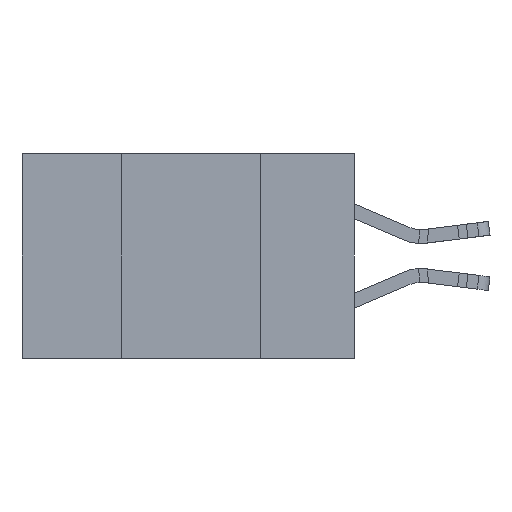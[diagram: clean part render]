
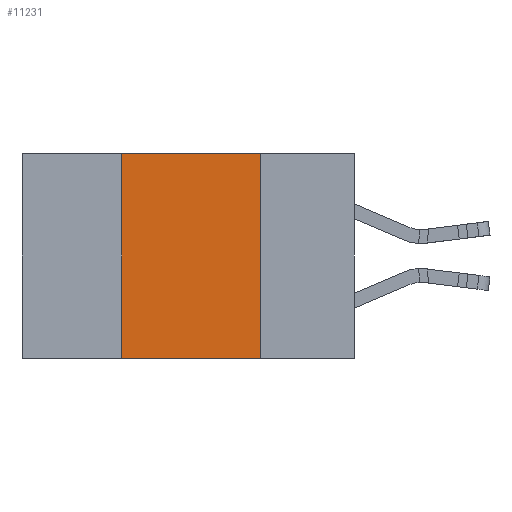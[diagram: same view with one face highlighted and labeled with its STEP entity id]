
A CAD part, left-side view. The second image highlights one B-rep face of the part: STEP entity #11231.
In plain terms, the highlighted planar face has unit normal (-1, 0, 0).
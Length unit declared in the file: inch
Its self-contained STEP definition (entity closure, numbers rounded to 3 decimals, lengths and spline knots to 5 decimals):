
#298 = ORIENTED_EDGE ( 'NONE', *, *, #9223, .T. ) ;
#369 = CARTESIAN_POINT ( 'NONE',  ( 0., 0.42, -0.37 ) ) ;
#645 = CARTESIAN_POINT ( 'NONE',  ( 0., 0.6, -0.37 ) ) ;
#2276 = VECTOR ( 'NONE', #17436, 39.37008 ) ;
#2547 = EDGE_CURVE ( 'NONE', #14172, #7647, #21391, .T. ) ;
#2698 = VERTEX_POINT ( 'NONE', #369 ) ;
#3927 = EDGE_CURVE ( 'NONE', #15790, #14172, #23972, .T. ) ;
#4659 = ORIENTED_EDGE ( 'NONE', *, *, #2547, .F. ) ;
#5021 = ORIENTED_EDGE ( 'NONE', *, *, #13485, .F. ) ;
#5457 = DIRECTION ( 'NONE',  ( 1., 0., 0. ) ) ;
#7014 = FACE_OUTER_BOUND ( 'NONE', #19034, .T. ) ;
#7462 = ORIENTED_EDGE ( 'NONE', *, *, #3927, .F. ) ;
#7647 = VERTEX_POINT ( 'NONE', #14133 ) ;
#9033 = LINE ( 'NONE', #645, #12947 ) ;
#9223 = EDGE_CURVE ( 'NONE', #2698, #7647, #9033, .T. ) ;
#11231 = ADVANCED_FACE ( 'NONE', ( #7014 ), #13076, .F. ) ;
#12184 = AXIS2_PLACEMENT_3D ( 'NONE', #18988, #5457, #16800 ) ;
#12947 = VECTOR ( 'NONE', #22443, 39.37008 ) ;
#13076 = PLANE ( 'NONE',  #12184 ) ;
#13485 = EDGE_CURVE ( 'NONE', #2698, #15790, #15013, .T. ) ;
#14133 = CARTESIAN_POINT ( 'NONE',  ( 0., 0.17, -0.37 ) ) ;
#14172 = VERTEX_POINT ( 'NONE', #25130 ) ;
#15013 = LINE ( 'NONE', #20903, #15773 ) ;
#15773 = VECTOR ( 'NONE', #21032, 39.37008 ) ;
#15790 = VERTEX_POINT ( 'NONE', #24601 ) ;
#16800 = DIRECTION ( 'NONE',  ( 0., 0., -1. ) ) ;
#17436 = DIRECTION ( 'NONE',  ( 0., 0., -1. ) ) ;
#17557 = CARTESIAN_POINT ( 'NONE',  ( 0., 0.17, -0.37 ) ) ;
#18054 = DIRECTION ( 'NONE',  ( 0., -1., 0. ) ) ;
#18988 = CARTESIAN_POINT ( 'NONE',  ( 0., 0.6, 0. ) ) ;
#19034 = EDGE_LOOP ( 'NONE', ( #4659, #7462, #5021, #298 ) ) ;
#20229 = CARTESIAN_POINT ( 'NONE',  ( 0., 0.6, 0. ) ) ;
#20623 = VECTOR ( 'NONE', #18054, 39.37008 ) ;
#20903 = CARTESIAN_POINT ( 'NONE',  ( 0., 0.42, -0.37 ) ) ;
#21032 = DIRECTION ( 'NONE',  ( 0., 0., 1. ) ) ;
#21391 = LINE ( 'NONE', #17557, #2276 ) ;
#22443 = DIRECTION ( 'NONE',  ( 0., -1., 0. ) ) ;
#23972 = LINE ( 'NONE', #20229, #20623 ) ;
#24601 = CARTESIAN_POINT ( 'NONE',  ( 0., 0.42, 0. ) ) ;
#25130 = CARTESIAN_POINT ( 'NONE',  ( 0., 0.17, 0. ) ) ;
